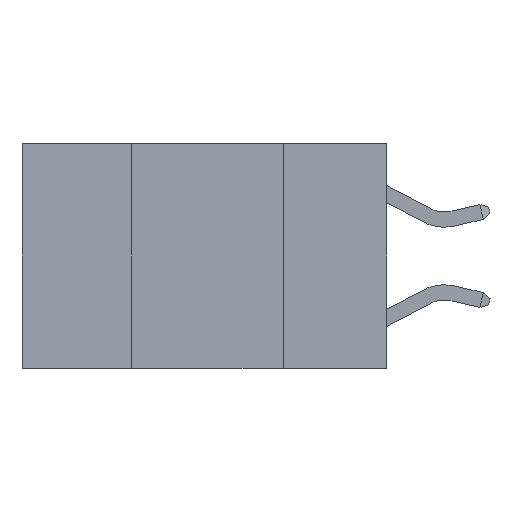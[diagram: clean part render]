
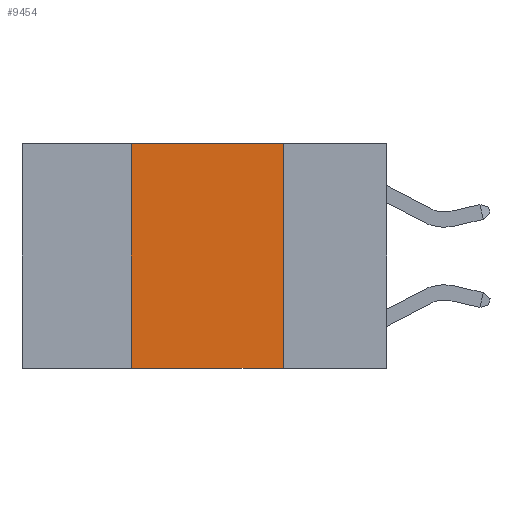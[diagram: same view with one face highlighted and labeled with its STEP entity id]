
A CAD part, left-side view. The second image highlights one B-rep face of the part: STEP entity #9454.
In plain terms, the highlighted planar face has unit normal (-1, 0, 0).
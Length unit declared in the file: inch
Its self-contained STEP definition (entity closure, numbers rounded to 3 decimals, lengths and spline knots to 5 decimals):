
#273 = DIRECTION ( 'NONE',  ( 0., -1., 0. ) ) ;
#437 = PLANE ( 'NONE',  #25487 ) ;
#736 = EDGE_CURVE ( 'NONE', #21829, #24599, #3561, .T. ) ;
#878 = CARTESIAN_POINT ( 'NONE',  ( 0., 0.42, 0. ) ) ;
#2292 = VECTOR ( 'NONE', #20358, 39.37008 ) ;
#2492 = CARTESIAN_POINT ( 'NONE',  ( 0., 0.17, 0. ) ) ;
#2562 = FACE_OUTER_BOUND ( 'NONE', #13166, .T. ) ;
#2646 = CARTESIAN_POINT ( 'NONE',  ( 0., 0.42, -0.37 ) ) ;
#3561 = LINE ( 'NONE', #10353, #2292 ) ;
#5371 = ORIENTED_EDGE ( 'NONE', *, *, #6862, .T. ) ;
#6862 = EDGE_CURVE ( 'NONE', #20275, #24599, #7873, .T. ) ;
#7873 = LINE ( 'NONE', #17871, #10582 ) ;
#9454 = ADVANCED_FACE ( 'NONE', ( #2562 ), #437, .F. ) ;
#10131 = CARTESIAN_POINT ( 'NONE',  ( 0., 0.6, 0. ) ) ;
#10205 = CARTESIAN_POINT ( 'NONE',  ( 0., 0.17, -0.37 ) ) ;
#10353 = CARTESIAN_POINT ( 'NONE',  ( 0., 0.17, 0. ) ) ;
#10582 = VECTOR ( 'NONE', #22734, 39.37008 ) ;
#13166 = EDGE_LOOP ( 'NONE', ( #29308, #29293, #28544, #5371 ) ) ;
#13507 = VECTOR ( 'NONE', #16050, 39.37008 ) ;
#16050 = DIRECTION ( 'NONE',  ( 0., 0., 1. ) ) ;
#16441 = CARTESIAN_POINT ( 'NONE',  ( 0., 0.42, 0. ) ) ;
#17871 = CARTESIAN_POINT ( 'NONE',  ( 0., 0.6, -0.37 ) ) ;
#20275 = VERTEX_POINT ( 'NONE', #2646 ) ;
#20358 = DIRECTION ( 'NONE',  ( 0., 0., -1. ) ) ;
#20439 = VERTEX_POINT ( 'NONE', #16441 ) ;
#21829 = VERTEX_POINT ( 'NONE', #2492 ) ;
#22710 = DIRECTION ( 'NONE',  ( 1., 0., 0. ) ) ;
#22734 = DIRECTION ( 'NONE',  ( 0., -1., 0. ) ) ;
#23613 = LINE ( 'NONE', #878, #13507 ) ;
#24335 = CARTESIAN_POINT ( 'NONE',  ( 0., 0.6, 0. ) ) ;
#24599 = VERTEX_POINT ( 'NONE', #10205 ) ;
#25487 = AXIS2_PLACEMENT_3D ( 'NONE', #10131, #22710, #29957 ) ;
#28544 = ORIENTED_EDGE ( 'NONE', *, *, #30182, .F. ) ;
#29293 = ORIENTED_EDGE ( 'NONE', *, *, #31397, .F. ) ;
#29308 = ORIENTED_EDGE ( 'NONE', *, *, #736, .F. ) ;
#29957 = DIRECTION ( 'NONE',  ( 0., 0., -1. ) ) ;
#30182 = EDGE_CURVE ( 'NONE', #20275, #20439, #23613, .T. ) ;
#31397 = EDGE_CURVE ( 'NONE', #20439, #21829, #31736, .T. ) ;
#31564 = VECTOR ( 'NONE', #273, 39.37008 ) ;
#31736 = LINE ( 'NONE', #24335, #31564 ) ;
